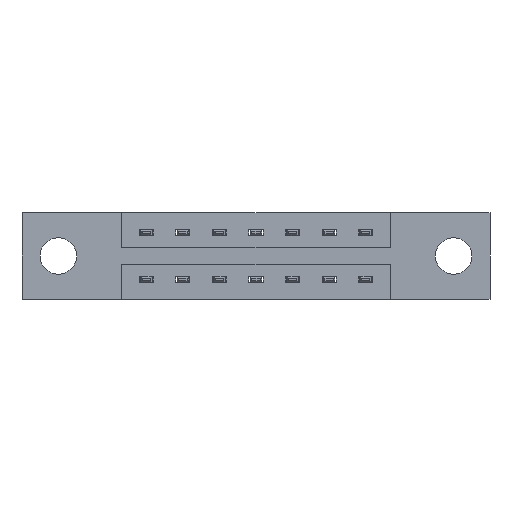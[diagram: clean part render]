
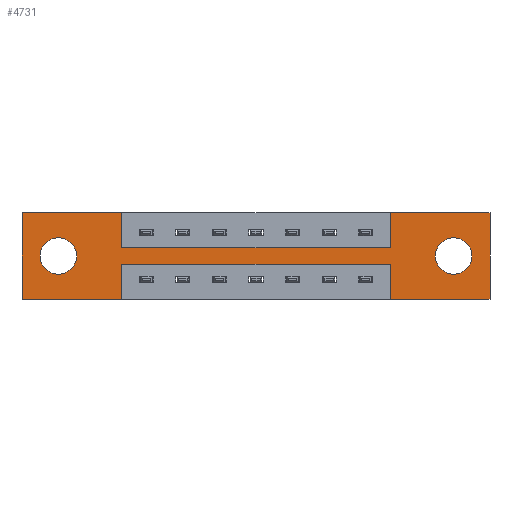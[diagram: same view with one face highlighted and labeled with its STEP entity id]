
A CAD part, front view. The second image highlights one B-rep face of the part: STEP entity #4731.
In plain terms, the highlighted planar face has unit normal (0, -1, 0).
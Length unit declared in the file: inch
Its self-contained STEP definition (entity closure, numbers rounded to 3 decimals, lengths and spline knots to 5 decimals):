
#125 = LINE ( 'NONE', #8029, #850 ) ;
#217 = LINE ( 'NONE', #7917, #9584 ) ;
#327 = DIRECTION ( 'NONE',  ( 0., 0., 1. ) ) ;
#353 = EDGE_CURVE ( 'NONE', #3093, #2192, #2773, .T. ) ;
#359 = ORIENTED_EDGE ( 'NONE', *, *, #7296, .F. ) ;
#363 = VECTOR ( 'NONE', #7981, 39.37008 ) ;
#375 = ORIENTED_EDGE ( 'NONE', *, *, #4501, .F. ) ;
#417 = VECTOR ( 'NONE', #3972, 39.37008 ) ;
#460 = CARTESIAN_POINT ( 'NONE',  ( 0., 0., 0. ) ) ;
#655 = LINE ( 'NONE', #6559, #417 ) ;
#837 = DIRECTION ( 'NONE',  ( 0., 0., -1. ) ) ;
#850 = VECTOR ( 'NONE', #6763, 39.37008 ) ;
#883 = EDGE_LOOP ( 'NONE', ( #1777, #7150 ) ) ;
#899 = EDGE_LOOP ( 'NONE', ( #8095, #1216 ) ) ;
#963 = VECTOR ( 'NONE', #6338, 39.37008 ) ;
#981 = DIRECTION ( 'NONE',  ( -1., 0., 0. ) ) ;
#1076 = VERTEX_POINT ( 'NONE', #7060 ) ;
#1080 = LINE ( 'NONE', #9577, #5155 ) ;
#1216 = ORIENTED_EDGE ( 'NONE', *, *, #3275, .T. ) ;
#1230 = ORIENTED_EDGE ( 'NONE', *, *, #2285, .F. ) ;
#1279 = VERTEX_POINT ( 'NONE', #6863 ) ;
#1428 = AXIS2_PLACEMENT_3D ( 'NONE', #8054, #6585, #6577 ) ;
#1500 = CARTESIAN_POINT ( 'NONE',  ( 0., 0., -0.37 ) ) ;
#1548 = VECTOR ( 'NONE', #3697, 39.37008 ) ;
#1600 = EDGE_LOOP ( 'NONE', ( #1230, #375, #9285, #5889, #8225, #359, #1789, #7640, #7653, #9628, #5823, #5364 ) ) ;
#1647 = VERTEX_POINT ( 'NONE', #8020 ) ;
#1669 = FACE_OUTER_BOUND ( 'NONE', #1600, .T. ) ;
#1716 = CARTESIAN_POINT ( 'NONE',  ( 1.843, 0., -0.185 ) ) ;
#1723 = DIRECTION ( 'NONE',  ( 0., 1., 0. ) ) ;
#1777 = ORIENTED_EDGE ( 'NONE', *, *, #7523, .T. ) ;
#1789 = ORIENTED_EDGE ( 'NONE', *, *, #353, .F. ) ;
#1810 = CARTESIAN_POINT ( 'NONE',  ( 1.573, 0., 0. ) ) ;
#1851 = DIRECTION ( 'NONE',  ( 0., 0., -1. ) ) ;
#1875 = DIRECTION ( 'NONE',  ( 0., 1., 0. ) ) ;
#1891 = CARTESIAN_POINT ( 'NONE',  ( 1.843, 0., -0.185 ) ) ;
#1992 = CIRCLE ( 'NONE', #2041, 0.078 ) ;
#2041 = AXIS2_PLACEMENT_3D ( 'NONE', #1891, #1875, #1851 ) ;
#2192 = VERTEX_POINT ( 'NONE', #4468 ) ;
#2249 = CARTESIAN_POINT ( 'NONE',  ( 0.155, 0., -0.107 ) ) ;
#2285 = EDGE_CURVE ( 'NONE', #5255, #3759, #125, .T. ) ;
#2309 = CARTESIAN_POINT ( 'NONE',  ( 1.998, 0., -0.37 ) ) ;
#2316 = LINE ( 'NONE', #8090, #8531 ) ;
#2374 = LINE ( 'NONE', #8576, #363 ) ;
#2526 = VECTOR ( 'NONE', #8974, 39.37008 ) ;
#2608 = VECTOR ( 'NONE', #8734, 39.37008 ) ;
#2668 = EDGE_CURVE ( 'NONE', #3487, #4299, #1080, .T. ) ;
#2709 = EDGE_CURVE ( 'NONE', #8466, #4336, #2847, .T. ) ;
#2749 = EDGE_CURVE ( 'NONE', #6035, #3093, #2374, .T. ) ;
#2773 = LINE ( 'NONE', #1810, #2526 ) ;
#2847 = LINE ( 'NONE', #8898, #2608 ) ;
#2906 = CARTESIAN_POINT ( 'NONE',  ( 0.425, 0., 0. ) ) ;
#2951 = EDGE_CURVE ( 'NONE', #7313, #7522, #7273, .T. ) ;
#3093 = VERTEX_POINT ( 'NONE', #8591 ) ;
#3166 = FACE_BOUND ( 'NONE', #883, .T. ) ;
#3225 = AXIS2_PLACEMENT_3D ( 'NONE', #1716, #1723, #837 ) ;
#3254 = VERTEX_POINT ( 'NONE', #4391 ) ;
#3275 = EDGE_CURVE ( 'NONE', #1076, #9692, #4315, .T. ) ;
#3487 = VERTEX_POINT ( 'NONE', #9574 ) ;
#3545 = CARTESIAN_POINT ( 'NONE',  ( 0.425, 0., -0.15 ) ) ;
#3573 = CARTESIAN_POINT ( 'NONE',  ( 0.425, 0., -0.22 ) ) ;
#3679 = CARTESIAN_POINT ( 'NONE',  ( 0., 0., -0.37 ) ) ;
#3697 = DIRECTION ( 'NONE',  ( -1., 0., 0. ) ) ;
#3759 = VERTEX_POINT ( 'NONE', #7787 ) ;
#3972 = DIRECTION ( 'NONE',  ( -1., 0., 0. ) ) ;
#3981 = CIRCLE ( 'NONE', #8932, 0.078 ) ;
#3994 = DIRECTION ( 'NONE',  ( 0., 0., 1. ) ) ;
#4037 = DIRECTION ( 'NONE',  ( 0., 1., 0. ) ) ;
#4049 = CARTESIAN_POINT ( 'NONE',  ( 0.155, 0., -0.185 ) ) ;
#4097 = AXIS2_PLACEMENT_3D ( 'NONE', #1500, #5181, #9551 ) ;
#4299 = VERTEX_POINT ( 'NONE', #2309 ) ;
#4315 = CIRCLE ( 'NONE', #1428, 0.078 ) ;
#4336 = VERTEX_POINT ( 'NONE', #5885 ) ;
#4391 = CARTESIAN_POINT ( 'NONE',  ( 1.843, 0., -0.107 ) ) ;
#4468 = CARTESIAN_POINT ( 'NONE',  ( 1.573, 0., 0. ) ) ;
#4501 = EDGE_CURVE ( 'NONE', #4336, #5255, #217, .T. ) ;
#4542 = EDGE_CURVE ( 'NONE', #3759, #1279, #9379, .T. ) ;
#4731 = ADVANCED_FACE ( 'NONE', ( #3166, #7475, #1669 ), #5994, .T. ) ;
#5155 = VECTOR ( 'NONE', #9200, 39.37008 ) ;
#5181 = DIRECTION ( 'NONE',  ( 0., -1., 0. ) ) ;
#5240 = CIRCLE ( 'NONE', #3225, 0.078 ) ;
#5255 = VERTEX_POINT ( 'NONE', #3573 ) ;
#5364 = ORIENTED_EDGE ( 'NONE', *, *, #4542, .F. ) ;
#5500 = EDGE_CURVE ( 'NONE', #7522, #6035, #2316, .T. ) ;
#5574 = CARTESIAN_POINT ( 'NONE',  ( 0., 0., 0. ) ) ;
#5654 = DIRECTION ( 'NONE',  ( 0., 0., -1. ) ) ;
#5696 = EDGE_CURVE ( 'NONE', #4299, #8466, #655, .T. ) ;
#5823 = ORIENTED_EDGE ( 'NONE', *, *, #8378, .F. ) ;
#5885 = CARTESIAN_POINT ( 'NONE',  ( 1.573, 0., -0.22 ) ) ;
#5889 = ORIENTED_EDGE ( 'NONE', *, *, #5696, .F. ) ;
#5994 = PLANE ( 'NONE',  #4097 ) ;
#6035 = VERTEX_POINT ( 'NONE', #3545 ) ;
#6338 = DIRECTION ( 'NONE',  ( 1., 0., 0. ) ) ;
#6559 = CARTESIAN_POINT ( 'NONE',  ( 0., 0., -0.37 ) ) ;
#6577 = DIRECTION ( 'NONE',  ( 0., 0., 1. ) ) ;
#6585 = DIRECTION ( 'NONE',  ( 0., 1., 0. ) ) ;
#6763 = DIRECTION ( 'NONE',  ( 0., 0., -1. ) ) ;
#6767 = CARTESIAN_POINT ( 'NONE',  ( 0., 0., 0. ) ) ;
#6863 = CARTESIAN_POINT ( 'NONE',  ( 0., 0., -0.37 ) ) ;
#6881 = VECTOR ( 'NONE', #327, 39.37008 ) ;
#7060 = CARTESIAN_POINT ( 'NONE',  ( 0.155, 0., -0.263 ) ) ;
#7119 = LINE ( 'NONE', #7213, #8760 ) ;
#7146 = DIRECTION ( 'NONE',  ( 1., 0., 0. ) ) ;
#7150 = ORIENTED_EDGE ( 'NONE', *, *, #8265, .T. ) ;
#7213 = CARTESIAN_POINT ( 'NONE',  ( 0., 0., 0. ) ) ;
#7273 = LINE ( 'NONE', #5574, #963 ) ;
#7296 = EDGE_CURVE ( 'NONE', #2192, #3487, #7119, .T. ) ;
#7313 = VERTEX_POINT ( 'NONE', #6767 ) ;
#7475 = FACE_BOUND ( 'NONE', #899, .T. ) ;
#7522 = VERTEX_POINT ( 'NONE', #2906 ) ;
#7523 = EDGE_CURVE ( 'NONE', #3254, #1647, #5240, .T. ) ;
#7640 = ORIENTED_EDGE ( 'NONE', *, *, #2749, .F. ) ;
#7653 = ORIENTED_EDGE ( 'NONE', *, *, #5500, .F. ) ;
#7787 = CARTESIAN_POINT ( 'NONE',  ( 0.425, 0., -0.37 ) ) ;
#7917 = CARTESIAN_POINT ( 'NONE',  ( 0.425, 0., -0.22 ) ) ;
#7981 = DIRECTION ( 'NONE',  ( 1., 0., 0. ) ) ;
#8020 = CARTESIAN_POINT ( 'NONE',  ( 1.843, 0., -0.263 ) ) ;
#8029 = CARTESIAN_POINT ( 'NONE',  ( 0.425, 0., -0.37 ) ) ;
#8054 = CARTESIAN_POINT ( 'NONE',  ( 0.155, 0., -0.185 ) ) ;
#8061 = EDGE_CURVE ( 'NONE', #9692, #1076, #3981, .T. ) ;
#8090 = CARTESIAN_POINT ( 'NONE',  ( 0.425, 0., 0. ) ) ;
#8095 = ORIENTED_EDGE ( 'NONE', *, *, #8061, .T. ) ;
#8225 = ORIENTED_EDGE ( 'NONE', *, *, #2668, .F. ) ;
#8265 = EDGE_CURVE ( 'NONE', #1647, #3254, #1992, .T. ) ;
#8378 = EDGE_CURVE ( 'NONE', #1279, #7313, #8749, .T. ) ;
#8466 = VERTEX_POINT ( 'NONE', #9633 ) ;
#8531 = VECTOR ( 'NONE', #5654, 39.37008 ) ;
#8576 = CARTESIAN_POINT ( 'NONE',  ( 0.425, 0., -0.15 ) ) ;
#8591 = CARTESIAN_POINT ( 'NONE',  ( 1.573, 0., -0.15 ) ) ;
#8734 = DIRECTION ( 'NONE',  ( 0., 0., 1. ) ) ;
#8749 = LINE ( 'NONE', #460, #6881 ) ;
#8760 = VECTOR ( 'NONE', #7146, 39.37008 ) ;
#8898 = CARTESIAN_POINT ( 'NONE',  ( 1.573, 0., -0.37 ) ) ;
#8932 = AXIS2_PLACEMENT_3D ( 'NONE', #4049, #4037, #3994 ) ;
#8974 = DIRECTION ( 'NONE',  ( 0., 0., 1. ) ) ;
#9200 = DIRECTION ( 'NONE',  ( 0., 0., -1. ) ) ;
#9285 = ORIENTED_EDGE ( 'NONE', *, *, #2709, .F. ) ;
#9379 = LINE ( 'NONE', #3679, #1548 ) ;
#9551 = DIRECTION ( 'NONE',  ( 0., 0., -1. ) ) ;
#9574 = CARTESIAN_POINT ( 'NONE',  ( 1.998, 0., 0. ) ) ;
#9577 = CARTESIAN_POINT ( 'NONE',  ( 1.998, 0., 0. ) ) ;
#9584 = VECTOR ( 'NONE', #981, 39.37008 ) ;
#9628 = ORIENTED_EDGE ( 'NONE', *, *, #2951, .F. ) ;
#9633 = CARTESIAN_POINT ( 'NONE',  ( 1.573, 0., -0.37 ) ) ;
#9692 = VERTEX_POINT ( 'NONE', #2249 ) ;
